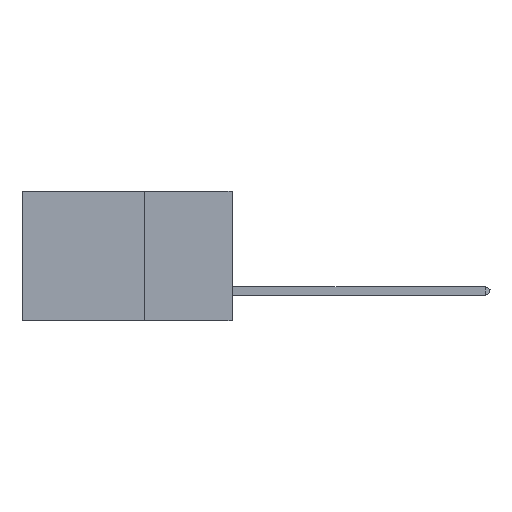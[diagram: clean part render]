
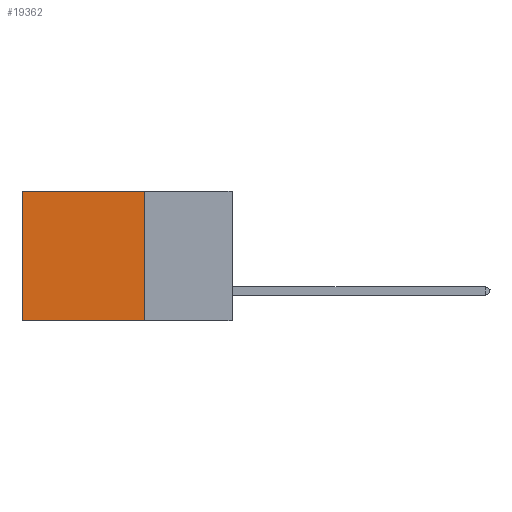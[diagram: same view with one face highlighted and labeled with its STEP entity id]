
A CAD part, left-side view. The second image highlights one B-rep face of the part: STEP entity #19362.
In plain terms, the highlighted planar face has unit normal (-1, 0, 0).
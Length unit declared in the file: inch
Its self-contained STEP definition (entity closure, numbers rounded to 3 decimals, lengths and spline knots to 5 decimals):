
#428 = ORIENTED_EDGE ( 'NONE', *, *, #11079, .T. ) ;
#836 = VECTOR ( 'NONE', #19343, 39.37008 ) ;
#1924 = CARTESIAN_POINT ( 'NONE',  ( 0.2875, 0.25, 0. ) ) ;
#2854 = LINE ( 'NONE', #24048, #18537 ) ;
#3129 = VECTOR ( 'NONE', #17540, 39.37008 ) ;
#4164 = DIRECTION ( 'NONE',  ( 0., 0., -1. ) ) ;
#4315 = EDGE_CURVE ( 'NONE', #26610, #4433, #21598, .T. ) ;
#4433 = VERTEX_POINT ( 'NONE', #11959 ) ;
#6306 = DIRECTION ( 'NONE',  ( 0., 1., 0. ) ) ;
#7315 = ORIENTED_EDGE ( 'NONE', *, *, #17286, .F. ) ;
#7507 = ORIENTED_EDGE ( 'NONE', *, *, #16585, .F. ) ;
#8059 = CARTESIAN_POINT ( 'NONE',  ( 0.2875, 0.25, 0. ) ) ;
#8425 = CARTESIAN_POINT ( 'NONE',  ( 0.2875, 0.25, 0. ) ) ;
#10340 = PLANE ( 'NONE',  #15290 ) ;
#11079 = EDGE_CURVE ( 'NONE', #17399, #26610, #17564, .T. ) ;
#11959 = CARTESIAN_POINT ( 'NONE',  ( 0.2875, 0.6, -0.37 ) ) ;
#13088 = VECTOR ( 'NONE', #14913, 39.37008 ) ;
#13262 = ORIENTED_EDGE ( 'NONE', *, *, #4315, .T. ) ;
#14913 = DIRECTION ( 'NONE',  ( 0., 1., 0. ) ) ;
#15232 = CARTESIAN_POINT ( 'NONE',  ( 0.2875, 0.6, 0. ) ) ;
#15290 = AXIS2_PLACEMENT_3D ( 'NONE', #25662, #25950, #4164 ) ;
#16585 = EDGE_CURVE ( 'NONE', #17399, #22963, #24081, .T. ) ;
#17286 = EDGE_CURVE ( 'NONE', #22963, #4433, #2854, .T. ) ;
#17399 = VERTEX_POINT ( 'NONE', #8425 ) ;
#17540 = DIRECTION ( 'NONE',  ( 0., 0., -1. ) ) ;
#17564 = LINE ( 'NONE', #1924, #13088 ) ;
#18537 = VECTOR ( 'NONE', #6306, 39.37008 ) ;
#19343 = DIRECTION ( 'NONE',  ( 0., 0., -1. ) ) ;
#19362 = ADVANCED_FACE ( 'NONE', ( #19826 ), #10340, .F. ) ;
#19826 = FACE_OUTER_BOUND ( 'NONE', #22977, .T. ) ;
#19987 = CARTESIAN_POINT ( 'NONE',  ( 0.2875, 0.6, 0. ) ) ;
#21598 = LINE ( 'NONE', #19987, #3129 ) ;
#22963 = VERTEX_POINT ( 'NONE', #24077 ) ;
#22977 = EDGE_LOOP ( 'NONE', ( #13262, #7315, #7507, #428 ) ) ;
#24048 = CARTESIAN_POINT ( 'NONE',  ( 0.2875, 0.25, -0.37 ) ) ;
#24077 = CARTESIAN_POINT ( 'NONE',  ( 0.2875, 0.25, -0.37 ) ) ;
#24081 = LINE ( 'NONE', #8059, #836 ) ;
#25662 = CARTESIAN_POINT ( 'NONE',  ( 0.2875, 0.25, 0. ) ) ;
#25950 = DIRECTION ( 'NONE',  ( 1., 0., 0. ) ) ;
#26610 = VERTEX_POINT ( 'NONE', #15232 ) ;
